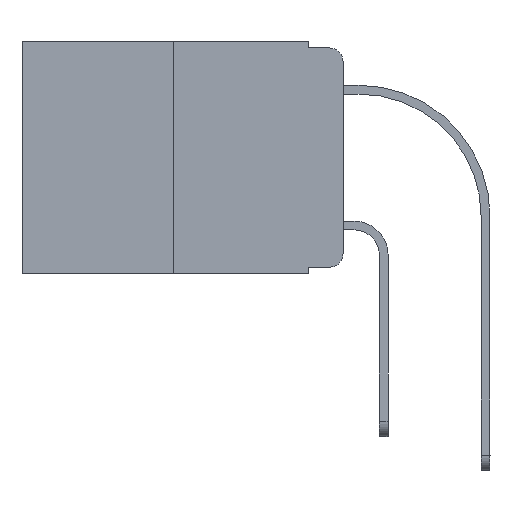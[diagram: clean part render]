
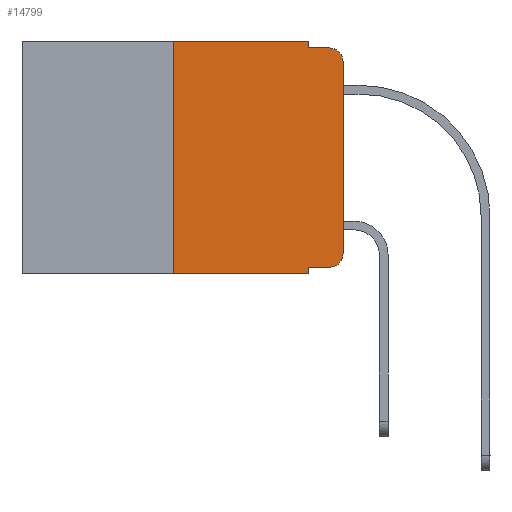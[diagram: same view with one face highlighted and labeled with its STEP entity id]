
A CAD part, left-side view. The second image highlights one B-rep face of the part: STEP entity #14799.
In plain terms, the highlighted planar face has unit normal (-1, 0, 0).
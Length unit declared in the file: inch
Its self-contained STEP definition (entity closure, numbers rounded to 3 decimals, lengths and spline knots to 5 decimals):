
#66 = EDGE_CURVE ( 'NONE', #19153, #3590, #10350, .T. ) ;
#135 = EDGE_CURVE ( 'NONE', #11051, #8740, #9773, .T. ) ;
#1519 = VECTOR ( 'NONE', #14721, 39.37008 ) ;
#1775 = DIRECTION ( 'NONE',  ( 0., -1., 0. ) ) ;
#1810 = CARTESIAN_POINT ( 'NONE',  ( 0., 0.02, -0.03 ) ) ;
#2647 = LINE ( 'NONE', #19174, #3049 ) ;
#2754 = VERTEX_POINT ( 'NONE', #23007 ) ;
#3049 = VECTOR ( 'NONE', #8179, 39.37008 ) ;
#3590 = VERTEX_POINT ( 'NONE', #9360 ) ;
#3603 = CIRCLE ( 'NONE', #4352, 0.02 ) ;
#3965 = EDGE_CURVE ( 'NONE', #3590, #4153, #22089, .T. ) ;
#4153 = VERTEX_POINT ( 'NONE', #15777 ) ;
#4352 = AXIS2_PLACEMENT_3D ( 'NONE', #1810, #19988, #5495 ) ;
#4498 = CARTESIAN_POINT ( 'NONE',  ( 0., 0.051, -0.333 ) ) ;
#4824 = CARTESIAN_POINT ( 'NONE',  ( 0., 0.02, -0.313 ) ) ;
#5495 = DIRECTION ( 'NONE',  ( 0., 0., -1. ) ) ;
#6047 = CARTESIAN_POINT ( 'NONE',  ( 0., 0., 0. ) ) ;
#6268 = ORIENTED_EDGE ( 'NONE', *, *, #66, .T. ) ;
#6327 = CARTESIAN_POINT ( 'NONE',  ( 0., 0.25, 0. ) ) ;
#7207 = VERTEX_POINT ( 'NONE', #4498 ) ;
#8100 = CARTESIAN_POINT ( 'NONE',  ( 0., 0.02, -0.01 ) ) ;
#8156 = DIRECTION ( 'NONE',  ( 0., -1., 0. ) ) ;
#8179 = DIRECTION ( 'NONE',  ( 0., 0., 1. ) ) ;
#8425 = VECTOR ( 'NONE', #9346, 39.37008 ) ;
#8740 = VERTEX_POINT ( 'NONE', #18636 ) ;
#9346 = DIRECTION ( 'NONE',  ( 0., -1., 0. ) ) ;
#9360 = CARTESIAN_POINT ( 'NONE',  ( 0., 0., -0.313 ) ) ;
#9516 = EDGE_CURVE ( 'NONE', #7207, #18814, #15959, .T. ) ;
#9678 = FACE_OUTER_BOUND ( 'NONE', #19224, .T. ) ;
#9773 = LINE ( 'NONE', #15258, #14544 ) ;
#9944 = LINE ( 'NONE', #23048, #18611 ) ;
#10039 = ORIENTED_EDGE ( 'NONE', *, *, #17033, .T. ) ;
#10350 = CIRCLE ( 'NONE', #19876, 0.02 ) ;
#10739 = CARTESIAN_POINT ( 'NONE',  ( 0., 0.02, -0.333 ) ) ;
#11042 = VECTOR ( 'NONE', #21976, 39.37008 ) ;
#11051 = VERTEX_POINT ( 'NONE', #22840 ) ;
#12592 = CARTESIAN_POINT ( 'NONE',  ( 0., 0.051, 0. ) ) ;
#13146 = LINE ( 'NONE', #13266, #1519 ) ;
#13234 = ORIENTED_EDGE ( 'NONE', *, *, #16922, .T. ) ;
#13266 = CARTESIAN_POINT ( 'NONE',  ( 0., 0.473, -0.343 ) ) ;
#13362 = PLANE ( 'NONE',  #15696 ) ;
#14230 = EDGE_CURVE ( 'NONE', #8740, #21421, #21873, .T. ) ;
#14544 = VECTOR ( 'NONE', #19101, 39.37008 ) ;
#14641 = EDGE_CURVE ( 'NONE', #21842, #11051, #21495, .T. ) ;
#14721 = DIRECTION ( 'NONE',  ( 0., -1., 0. ) ) ;
#14799 = ADVANCED_FACE ( 'NONE', ( #9678 ), #13362, .F. ) ;
#14804 = DIRECTION ( 'NONE',  ( 1., 0., 0. ) ) ;
#15258 = CARTESIAN_POINT ( 'NONE',  ( 0., 0.051, 0. ) ) ;
#15280 = CARTESIAN_POINT ( 'NONE',  ( 0., 0.473, 0. ) ) ;
#15696 = AXIS2_PLACEMENT_3D ( 'NONE', #15280, #14804, #20299 ) ;
#15777 = CARTESIAN_POINT ( 'NONE',  ( 0., 0., -0.03 ) ) ;
#15941 = VECTOR ( 'NONE', #18113, 39.37008 ) ;
#15959 = LINE ( 'NONE', #12592, #15941 ) ;
#16133 = ORIENTED_EDGE ( 'NONE', *, *, #17267, .T. ) ;
#16589 = ORIENTED_EDGE ( 'NONE', *, *, #14230, .F. ) ;
#16913 = ORIENTED_EDGE ( 'NONE', *, *, #21816, .F. ) ;
#16922 = EDGE_CURVE ( 'NONE', #4153, #21421, #3603, .T. ) ;
#17033 = EDGE_CURVE ( 'NONE', #2754, #18814, #13146, .T. ) ;
#17267 = EDGE_CURVE ( 'NONE', #7207, #19153, #9944, .T. ) ;
#17422 = DIRECTION ( 'NONE',  ( 0., 0., -1. ) ) ;
#17484 = ORIENTED_EDGE ( 'NONE', *, *, #9516, .F. ) ;
#17596 = VECTOR ( 'NONE', #1775, 39.37008 ) ;
#18058 = CARTESIAN_POINT ( 'NONE',  ( 0., 0.473, 0. ) ) ;
#18113 = DIRECTION ( 'NONE',  ( 0., 0., -1. ) ) ;
#18611 = VECTOR ( 'NONE', #8156, 39.37008 ) ;
#18636 = CARTESIAN_POINT ( 'NONE',  ( 0., 0.051, -0.01 ) ) ;
#18814 = VERTEX_POINT ( 'NONE', #22433 ) ;
#19101 = DIRECTION ( 'NONE',  ( 0., 0., -1. ) ) ;
#19153 = VERTEX_POINT ( 'NONE', #10739 ) ;
#19174 = CARTESIAN_POINT ( 'NONE',  ( 0., 0.25, 0. ) ) ;
#19224 = EDGE_LOOP ( 'NONE', ( #21488, #13234, #16589, #22415, #23371, #16913, #10039, #17484, #16133, #6268 ) ) ;
#19876 = AXIS2_PLACEMENT_3D ( 'NONE', #4824, #21220, #17422 ) ;
#19988 = DIRECTION ( 'NONE',  ( -1., 0., 0. ) ) ;
#20299 = DIRECTION ( 'NONE',  ( 0., 0., -1. ) ) ;
#21220 = DIRECTION ( 'NONE',  ( -1., 0., 0. ) ) ;
#21421 = VERTEX_POINT ( 'NONE', #8100 ) ;
#21488 = ORIENTED_EDGE ( 'NONE', *, *, #3965, .T. ) ;
#21495 = LINE ( 'NONE', #18058, #17596 ) ;
#21816 = EDGE_CURVE ( 'NONE', #2754, #21842, #2647, .T. ) ;
#21842 = VERTEX_POINT ( 'NONE', #6327 ) ;
#21873 = LINE ( 'NONE', #21981, #8425 ) ;
#21976 = DIRECTION ( 'NONE',  ( 0., 0., 1. ) ) ;
#21981 = CARTESIAN_POINT ( 'NONE',  ( 0., 0.051, -0.01 ) ) ;
#22089 = LINE ( 'NONE', #6047, #11042 ) ;
#22415 = ORIENTED_EDGE ( 'NONE', *, *, #135, .F. ) ;
#22433 = CARTESIAN_POINT ( 'NONE',  ( 0., 0.051, -0.343 ) ) ;
#22840 = CARTESIAN_POINT ( 'NONE',  ( 0., 0.051, 0. ) ) ;
#23007 = CARTESIAN_POINT ( 'NONE',  ( 0., 0.25, -0.343 ) ) ;
#23048 = CARTESIAN_POINT ( 'NONE',  ( 0., 0.051, -0.333 ) ) ;
#23371 = ORIENTED_EDGE ( 'NONE', *, *, #14641, .F. ) ;
